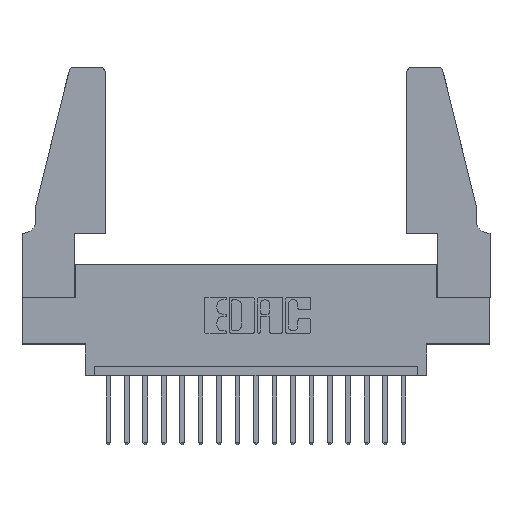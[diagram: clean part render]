
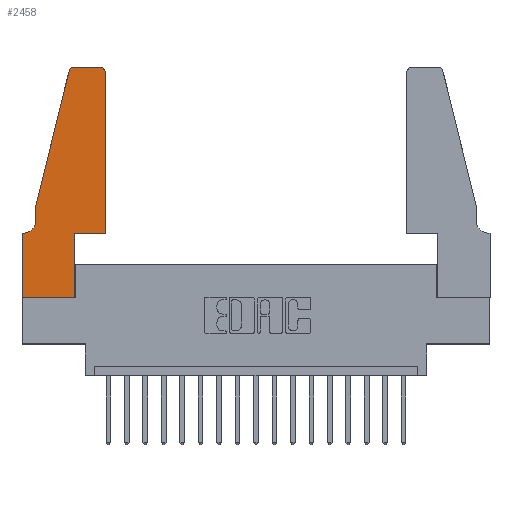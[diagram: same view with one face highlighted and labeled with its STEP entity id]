
A CAD part, top view. The second image highlights one B-rep face of the part: STEP entity #2458.
In plain terms, the highlighted planar face has unit normal (0, 0, 1).
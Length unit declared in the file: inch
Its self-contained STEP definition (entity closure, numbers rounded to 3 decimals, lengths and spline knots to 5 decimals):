
#409 = PLANE ( 'NONE',  #9984 ) ;
#600 = ORIENTED_EDGE ( 'NONE', *, *, #16727, .T. ) ;
#686 = CIRCLE ( 'NONE', #17983, 0.03 ) ;
#721 = VERTEX_POINT ( 'NONE', #12348 ) ;
#755 = ORIENTED_EDGE ( 'NONE', *, *, #9689, .T. ) ;
#859 = CARTESIAN_POINT ( 'NONE',  ( 0.284, 1.22, 0.37 ) ) ;
#1081 = CARTESIAN_POINT ( 'NONE',  ( 0.4205, 1.22, 0.37 ) ) ;
#1522 = VERTEX_POINT ( 'NONE', #18325 ) ;
#1795 = CARTESIAN_POINT ( 'NONE',  ( 0., 0.35, 0.37 ) ) ;
#2079 = CARTESIAN_POINT ( 'NONE',  ( 0.0755, 0.5, 0.37 ) ) ;
#2261 = VERTEX_POINT ( 'NONE', #14450 ) ;
#2458 = ADVANCED_FACE ( 'NONE', ( #9390 ), #409, .T. ) ;
#2473 = VECTOR ( 'NONE', #12251, 39.37008 ) ;
#2556 = ORIENTED_EDGE ( 'NONE', *, *, #7002, .T. ) ;
#3228 = DIRECTION ( 'NONE',  ( 1., 0., 0. ) ) ;
#3232 = DIRECTION ( 'NONE',  ( -1., 0., 0. ) ) ;
#3290 = DIRECTION ( 'NONE',  ( 0., 0., 1. ) ) ;
#3608 = CIRCLE ( 'NONE', #17741, 0.07 ) ;
#3668 = EDGE_CURVE ( 'NONE', #4289, #1522, #7557, .T. ) ;
#3850 = LINE ( 'NONE', #8391, #8360 ) ;
#3909 = EDGE_CURVE ( 'NONE', #2261, #5829, #17966, .T. ) ;
#4281 = CARTESIAN_POINT ( 'NONE',  ( 0.0755, 0.35, 0.37 ) ) ;
#4289 = VERTEX_POINT ( 'NONE', #14590 ) ;
#4737 = DIRECTION ( 'NONE',  ( 0., 0., -1. ) ) ;
#4847 = DIRECTION ( 'NONE',  ( 0., -1., 0. ) ) ;
#4905 = EDGE_CURVE ( 'NONE', #9345, #18394, #9763, .T. ) ;
#5485 = VECTOR ( 'NONE', #15621, 39.37008 ) ;
#5829 = VERTEX_POINT ( 'NONE', #8942 ) ;
#5919 = CARTESIAN_POINT ( 'NONE',  ( 0.0055, 0.35, 0.37 ) ) ;
#6094 = ORIENTED_EDGE ( 'NONE', *, *, #17250, .T. ) ;
#6246 = ORIENTED_EDGE ( 'NONE', *, *, #7297, .T. ) ;
#6561 = LINE ( 'NONE', #13800, #18101 ) ;
#6571 = ORIENTED_EDGE ( 'NONE', *, *, #15311, .T. ) ;
#6655 = DIRECTION ( 'NONE',  ( 0., 0., 1. ) ) ;
#6997 = DIRECTION ( 'NONE',  ( -0.239, -0.971, 0. ) ) ;
#7002 = EDGE_CURVE ( 'NONE', #5829, #17023, #3608, .T. ) ;
#7297 = EDGE_CURVE ( 'NONE', #7638, #9345, #686, .T. ) ;
#7557 = LINE ( 'NONE', #14566, #16185 ) ;
#7638 = VERTEX_POINT ( 'NONE', #11987 ) ;
#7741 = LINE ( 'NONE', #9697, #5485 ) ;
#8360 = VECTOR ( 'NONE', #6997, 39.37008 ) ;
#8381 = DIRECTION ( 'NONE',  ( 0., 0., 1. ) ) ;
#8391 = CARTESIAN_POINT ( 'NONE',  ( 0.0755, 0.5, 0.37 ) ) ;
#8794 = CARTESIAN_POINT ( 'NONE',  ( 0.4205, 1.25, 0.37 ) ) ;
#8942 = CARTESIAN_POINT ( 'NONE',  ( 0.0755, 0.42, 0.37 ) ) ;
#9345 = VERTEX_POINT ( 'NONE', #8794 ) ;
#9390 = FACE_OUTER_BOUND ( 'NONE', #17616, .T. ) ;
#9689 = EDGE_CURVE ( 'NONE', #11723, #2261, #3850, .T. ) ;
#9697 = CARTESIAN_POINT ( 'NONE',  ( 0.4505, 0.35, 0.37 ) ) ;
#9763 = LINE ( 'NONE', #15866, #17510 ) ;
#9984 = AXIS2_PLACEMENT_3D ( 'NONE', #1795, #3290, #3228 ) ;
#10214 = EDGE_CURVE ( 'NONE', #18394, #11723, #11441, .T. ) ;
#10284 = CARTESIAN_POINT ( 'NONE',  ( 0., 0., 0.37 ) ) ;
#10966 = EDGE_CURVE ( 'NONE', #12132, #4289, #16517, .T. ) ;
#10970 = DIRECTION ( 'NONE',  ( 0., 1., 0. ) ) ;
#11022 = CARTESIAN_POINT ( 'NONE',  ( 0.2865, 0.35, 0.37 ) ) ;
#11062 = LINE ( 'NONE', #4281, #14588 ) ;
#11093 = DIRECTION ( 'NONE',  ( 1., 0., 0. ) ) ;
#11441 = CIRCLE ( 'NONE', #16110, 0.03 ) ;
#11667 = DIRECTION ( 'NONE',  ( -1., 0., 0. ) ) ;
#11723 = VERTEX_POINT ( 'NONE', #17592 ) ;
#11863 = CARTESIAN_POINT ( 'NONE',  ( 0.284, 1.25, 0.37 ) ) ;
#11987 = CARTESIAN_POINT ( 'NONE',  ( 0.4505, 1.22, 0.37 ) ) ;
#12035 = DIRECTION ( 'NONE',  ( 0., -1., 0. ) ) ;
#12132 = VERTEX_POINT ( 'NONE', #13550 ) ;
#12251 = DIRECTION ( 'NONE',  ( 0., 1., 0. ) ) ;
#12310 = VERTEX_POINT ( 'NONE', #11022 ) ;
#12348 = CARTESIAN_POINT ( 'NONE',  ( 0.4505, 0.35, 0.37 ) ) ;
#12549 = ORIENTED_EDGE ( 'NONE', *, *, #3909, .T. ) ;
#12974 = CARTESIAN_POINT ( 'NONE',  ( 0.0055, 0.42, 0.37 ) ) ;
#13550 = CARTESIAN_POINT ( 'NONE',  ( 0., 0.35, 0.37 ) ) ;
#13762 = DIRECTION ( 'NONE',  ( 1., 0., 0. ) ) ;
#13800 = CARTESIAN_POINT ( 'NONE',  ( 0.4505, 0.35, 0.37 ) ) ;
#14057 = ORIENTED_EDGE ( 'NONE', *, *, #4905, .T. ) ;
#14210 = ORIENTED_EDGE ( 'NONE', *, *, #10966, .T. ) ;
#14450 = CARTESIAN_POINT ( 'NONE',  ( 0.0755, 0.5, 0.37 ) ) ;
#14566 = CARTESIAN_POINT ( 'NONE',  ( 0., 0., 0.37 ) ) ;
#14588 = VECTOR ( 'NONE', #11667, 39.37008 ) ;
#14590 = CARTESIAN_POINT ( 'NONE',  ( 0., 0., 0.37 ) ) ;
#14707 = ORIENTED_EDGE ( 'NONE', *, *, #15510, .T. ) ;
#14709 = VECTOR ( 'NONE', #4847, 39.37008 ) ;
#15311 = EDGE_CURVE ( 'NONE', #12310, #721, #7741, .T. ) ;
#15510 = EDGE_CURVE ( 'NONE', #17023, #12132, #11062, .T. ) ;
#15621 = DIRECTION ( 'NONE',  ( 1., 0., 0. ) ) ;
#15866 = CARTESIAN_POINT ( 'NONE',  ( 0.2605, 1.25, 0.37 ) ) ;
#15891 = CARTESIAN_POINT ( 'NONE',  ( 0.2865, 0.35, 0.37 ) ) ;
#16110 = AXIS2_PLACEMENT_3D ( 'NONE', #859, #6655, #13762 ) ;
#16125 = DIRECTION ( 'NONE',  ( -1., 0., 0. ) ) ;
#16185 = VECTOR ( 'NONE', #17184, 39.37008 ) ;
#16241 = ORIENTED_EDGE ( 'NONE', *, *, #10214, .T. ) ;
#16517 = LINE ( 'NONE', #10284, #14709 ) ;
#16628 = VECTOR ( 'NONE', #12035, 39.37008 ) ;
#16727 = EDGE_CURVE ( 'NONE', #721, #7638, #6561, .T. ) ;
#16978 = LINE ( 'NONE', #15891, #2473 ) ;
#17023 = VERTEX_POINT ( 'NONE', #5919 ) ;
#17184 = DIRECTION ( 'NONE',  ( 1., 0., 0. ) ) ;
#17250 = EDGE_CURVE ( 'NONE', #1522, #12310, #16978, .T. ) ;
#17510 = VECTOR ( 'NONE', #16125, 39.37008 ) ;
#17592 = CARTESIAN_POINT ( 'NONE',  ( 0.25487, 1.22718, 0.37 ) ) ;
#17616 = EDGE_LOOP ( 'NONE', ( #14057, #16241, #755, #12549, #2556, #14707, #14210, #17867, #6094, #6571, #600, #6246 ) ) ;
#17741 = AXIS2_PLACEMENT_3D ( 'NONE', #12974, #4737, #3232 ) ;
#17867 = ORIENTED_EDGE ( 'NONE', *, *, #3668, .T. ) ;
#17966 = LINE ( 'NONE', #2079, #16628 ) ;
#17983 = AXIS2_PLACEMENT_3D ( 'NONE', #1081, #8381, #11093 ) ;
#18101 = VECTOR ( 'NONE', #10970, 39.37008 ) ;
#18325 = CARTESIAN_POINT ( 'NONE',  ( 0.2865, 0., 0.37 ) ) ;
#18394 = VERTEX_POINT ( 'NONE', #11863 ) ;
